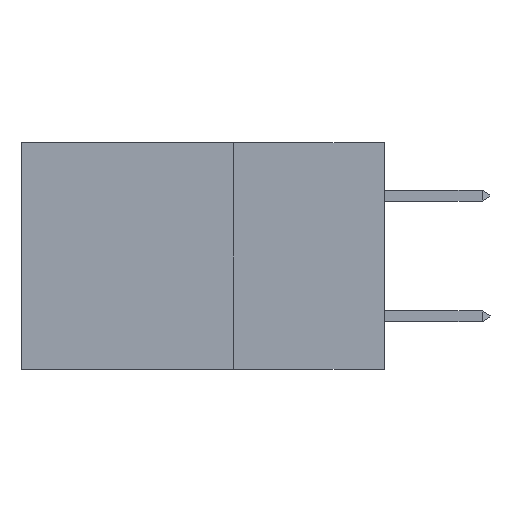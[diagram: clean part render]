
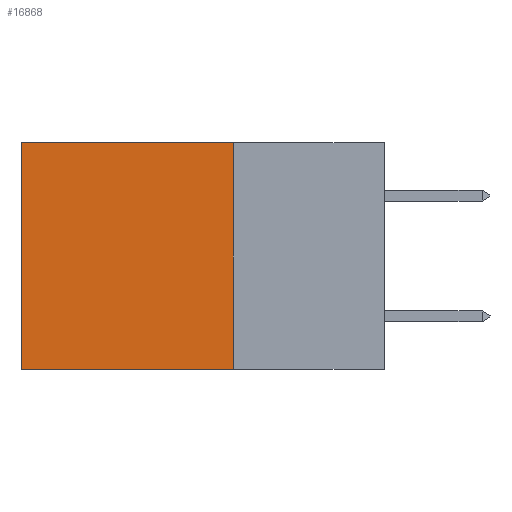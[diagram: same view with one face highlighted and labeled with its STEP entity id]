
A CAD part, left-side view. The second image highlights one B-rep face of the part: STEP entity #16868.
In plain terms, the highlighted planar face has unit normal (-1, 0, 0).
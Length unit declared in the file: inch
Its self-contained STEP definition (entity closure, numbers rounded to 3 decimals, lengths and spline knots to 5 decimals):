
#512 = VECTOR ( 'NONE', #8515, 39.37008 ) ;
#704 = AXIS2_PLACEMENT_3D ( 'NONE', #955, #1195, #1241 ) ;
#955 = CARTESIAN_POINT ( 'NONE',  ( 0.2875, 0.25, -0.375 ) ) ;
#1195 = DIRECTION ( 'NONE',  ( 1., 0., 0. ) ) ;
#1241 = DIRECTION ( 'NONE',  ( 0., 0., -1. ) ) ;
#1730 = ORIENTED_EDGE ( 'NONE', *, *, #5087, .F. ) ;
#2343 = ORIENTED_EDGE ( 'NONE', *, *, #13145, .F. ) ;
#2672 = VECTOR ( 'NONE', #15292, 39.37008 ) ;
#2891 = CARTESIAN_POINT ( 'NONE',  ( 0.2875, 0.6, -0.375 ) ) ;
#3182 = LINE ( 'NONE', #11884, #13251 ) ;
#4331 = VERTEX_POINT ( 'NONE', #16026 ) ;
#4623 = LINE ( 'NONE', #15000, #512 ) ;
#5087 = EDGE_CURVE ( 'NONE', #4331, #11523, #4623, .T. ) ;
#5462 = CARTESIAN_POINT ( 'NONE',  ( 0.2875, 0.25, 0. ) ) ;
#6113 = VERTEX_POINT ( 'NONE', #9223 ) ;
#6159 = LINE ( 'NONE', #12761, #2672 ) ;
#6166 = PLANE ( 'NONE',  #704 ) ;
#7194 = EDGE_LOOP ( 'NONE', ( #8628, #1730, #2343, #16642 ) ) ;
#7660 = LINE ( 'NONE', #9750, #15477 ) ;
#7863 = VERTEX_POINT ( 'NONE', #5462 ) ;
#7939 = EDGE_CURVE ( 'NONE', #7863, #6113, #6159, .T. ) ;
#8515 = DIRECTION ( 'NONE',  ( 0., 1., 0. ) ) ;
#8628 = ORIENTED_EDGE ( 'NONE', *, *, #13950, .T. ) ;
#9223 = CARTESIAN_POINT ( 'NONE',  ( 0.2875, 0.6, 0. ) ) ;
#9750 = CARTESIAN_POINT ( 'NONE',  ( 0.2875, 0.6, -0.375 ) ) ;
#10481 = FACE_OUTER_BOUND ( 'NONE', #7194, .T. ) ;
#11523 = VERTEX_POINT ( 'NONE', #2891 ) ;
#11884 = CARTESIAN_POINT ( 'NONE',  ( 0.2875, 0.25, -0.375 ) ) ;
#12761 = CARTESIAN_POINT ( 'NONE',  ( 0.2875, 0.25, 0. ) ) ;
#13145 = EDGE_CURVE ( 'NONE', #7863, #4331, #3182, .T. ) ;
#13251 = VECTOR ( 'NONE', #14517, 39.37008 ) ;
#13950 = EDGE_CURVE ( 'NONE', #6113, #11523, #7660, .T. ) ;
#14517 = DIRECTION ( 'NONE',  ( 0., 0., -1. ) ) ;
#15000 = CARTESIAN_POINT ( 'NONE',  ( 0.2875, 0.25, -0.375 ) ) ;
#15292 = DIRECTION ( 'NONE',  ( 0., 1., 0. ) ) ;
#15477 = VECTOR ( 'NONE', #16376, 39.37008 ) ;
#16026 = CARTESIAN_POINT ( 'NONE',  ( 0.2875, 0.25, -0.375 ) ) ;
#16376 = DIRECTION ( 'NONE',  ( 0., 0., -1. ) ) ;
#16642 = ORIENTED_EDGE ( 'NONE', *, *, #7939, .T. ) ;
#16868 = ADVANCED_FACE ( 'NONE', ( #10481 ), #6166, .F. ) ;
